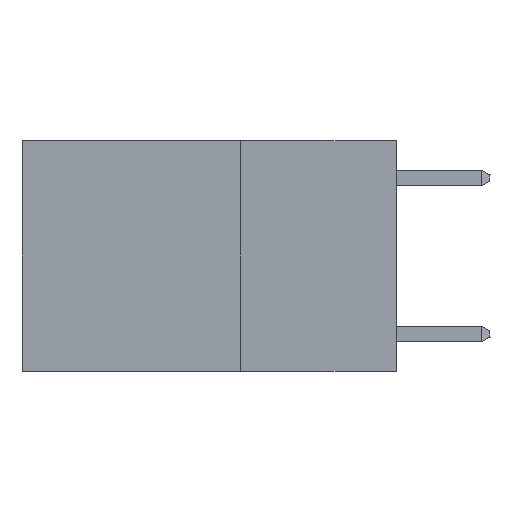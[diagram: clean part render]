
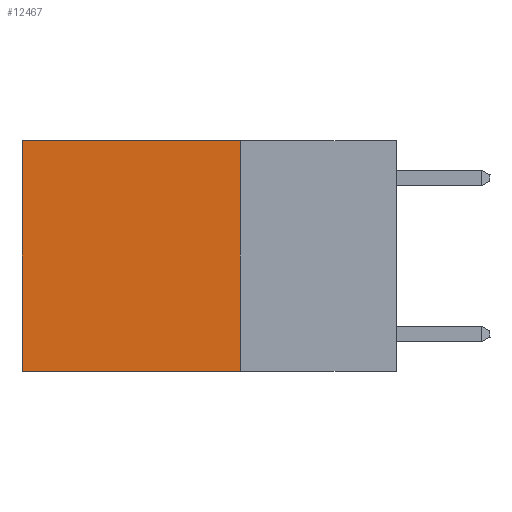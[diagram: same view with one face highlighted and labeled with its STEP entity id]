
A CAD part, left-side view. The second image highlights one B-rep face of the part: STEP entity #12467.
In plain terms, the highlighted planar face has unit normal (-1, 0, 0).
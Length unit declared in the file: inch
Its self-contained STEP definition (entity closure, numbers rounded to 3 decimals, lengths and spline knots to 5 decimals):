
#1267 = CARTESIAN_POINT ( 'NONE',  ( 0.2625, 0.6, 0. ) ) ;
#2984 = DIRECTION ( 'NONE',  ( 0., 0., -1. ) ) ;
#3994 = VERTEX_POINT ( 'NONE', #21386 ) ;
#4379 = EDGE_LOOP ( 'NONE', ( #4636, #16312, #9067, #12705 ) ) ;
#4509 = VERTEX_POINT ( 'NONE', #19597 ) ;
#4636 = ORIENTED_EDGE ( 'NONE', *, *, #18263, .T. ) ;
#5160 = CARTESIAN_POINT ( 'NONE',  ( 0.2625, 0.25, -0.37 ) ) ;
#5825 = DIRECTION ( 'NONE',  ( 0., 0., -1. ) ) ;
#6433 = EDGE_CURVE ( 'NONE', #3994, #16588, #13946, .T. ) ;
#6511 = DIRECTION ( 'NONE',  ( 0., 0., -1. ) ) ;
#6720 = EDGE_CURVE ( 'NONE', #3994, #14807, #14979, .T. ) ;
#6797 = VECTOR ( 'NONE', #12240, 39.37008 ) ;
#9067 = ORIENTED_EDGE ( 'NONE', *, *, #6433, .F. ) ;
#9857 = CARTESIAN_POINT ( 'NONE',  ( 0.2625, 0.25, 0. ) ) ;
#10606 = VECTOR ( 'NONE', #20322, 39.37008 ) ;
#10689 = CARTESIAN_POINT ( 'NONE',  ( 0.2625, 0.6, 0. ) ) ;
#10848 = LINE ( 'NONE', #5160, #6797 ) ;
#10936 = CARTESIAN_POINT ( 'NONE',  ( 0.2625, 0.25, 0. ) ) ;
#11190 = AXIS2_PLACEMENT_3D ( 'NONE', #10936, #18028, #5825 ) ;
#11274 = PLANE ( 'NONE',  #11190 ) ;
#11946 = EDGE_CURVE ( 'NONE', #16588, #4509, #10848, .T. ) ;
#12240 = DIRECTION ( 'NONE',  ( 0., 1., 0. ) ) ;
#12413 = CARTESIAN_POINT ( 'NONE',  ( 0.2625, 0.25, -0.37 ) ) ;
#12467 = ADVANCED_FACE ( 'NONE', ( #12675 ), #11274, .F. ) ;
#12675 = FACE_OUTER_BOUND ( 'NONE', #4379, .T. ) ;
#12705 = ORIENTED_EDGE ( 'NONE', *, *, #6720, .T. ) ;
#13946 = LINE ( 'NONE', #20696, #17542 ) ;
#14807 = VERTEX_POINT ( 'NONE', #10689 ) ;
#14979 = LINE ( 'NONE', #9857, #10606 ) ;
#16312 = ORIENTED_EDGE ( 'NONE', *, *, #11946, .F. ) ;
#16317 = VECTOR ( 'NONE', #2984, 39.37008 ) ;
#16588 = VERTEX_POINT ( 'NONE', #12413 ) ;
#17542 = VECTOR ( 'NONE', #6511, 39.37008 ) ;
#18028 = DIRECTION ( 'NONE',  ( 1., 0., 0. ) ) ;
#18263 = EDGE_CURVE ( 'NONE', #14807, #4509, #22419, .T. ) ;
#19597 = CARTESIAN_POINT ( 'NONE',  ( 0.2625, 0.6, -0.37 ) ) ;
#20322 = DIRECTION ( 'NONE',  ( 0., 1., 0. ) ) ;
#20696 = CARTESIAN_POINT ( 'NONE',  ( 0.2625, 0.25, 0. ) ) ;
#21386 = CARTESIAN_POINT ( 'NONE',  ( 0.2625, 0.25, 0. ) ) ;
#22419 = LINE ( 'NONE', #1267, #16317 ) ;
